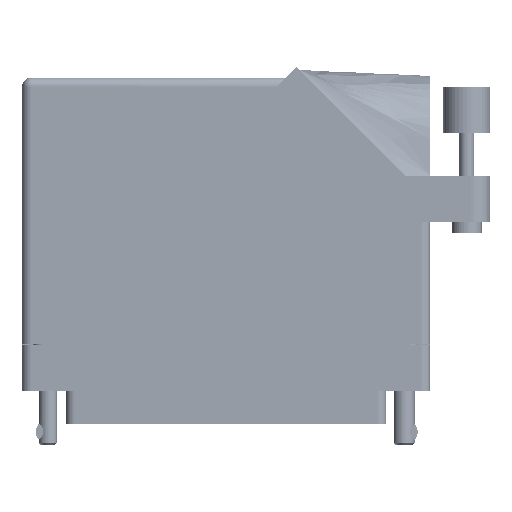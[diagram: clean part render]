
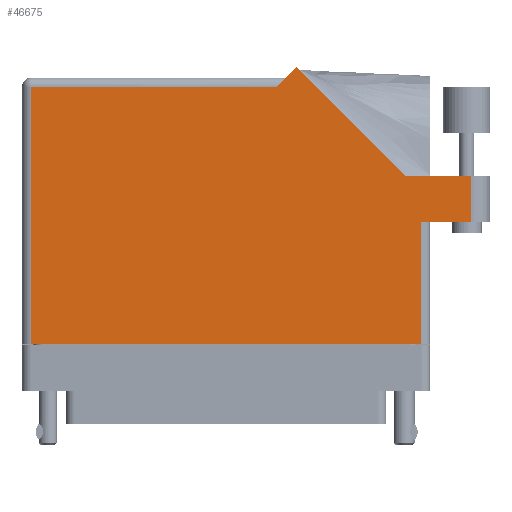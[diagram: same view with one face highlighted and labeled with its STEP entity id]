
A CAD part, front view. The second image highlights one B-rep face of the part: STEP entity #46675.
In plain terms, the highlighted face is planar.
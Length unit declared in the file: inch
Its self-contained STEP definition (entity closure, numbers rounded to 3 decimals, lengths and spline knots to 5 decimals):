
#30 = EDGE_CURVE ( 'NONE', #46746, #72187, #80173, .T. ) ;
#500 = EDGE_CURVE ( 'NONE', #21925, #56165, #10249, .T. ) ;
#1463 = CARTESIAN_POINT ( 'NONE',  ( -1.359, -0.1, 0.617 ) ) ;
#1577 = CARTESIAN_POINT ( 'NONE',  ( 0.399, 1.675, 0.617 ) ) ;
#2325 = DIRECTION ( 'NONE',  ( 1., 0., 0. ) ) ;
#2391 = CARTESIAN_POINT ( 'NONE',  ( 1.297, 0.715, 0.617 ) ) ;
#3229 = ORIENTED_EDGE ( 'NONE', *, *, #41724, .T. ) ;
#4679 = EDGE_CURVE ( 'NONE', #58465, #71421, #20613, .T. ) ;
#4954 = DIRECTION ( 'NONE',  ( 0., 1., 0. ) ) ;
#5821 = VECTOR ( 'NONE', #79149, 39.37008 ) ;
#6263 = DIRECTION ( 'NONE',  ( -1., 0., 0. ) ) ;
#9476 = PLANE ( 'NONE',  #22034 ) ;
#10249 = LINE ( 'NONE', #1463, #49826 ) ;
#11422 = CARTESIAN_POINT ( 'NONE',  ( -1.297, -0.1, 0.617 ) ) ;
#12130 = VECTOR ( 'NONE', #2325, 39.37008 ) ;
#12476 = CARTESIAN_POINT ( 'NONE',  ( 0.46971, 1.74571, 0.617 ) ) ;
#13965 = DIRECTION ( 'NONE',  ( 1., 0., 0. ) ) ;
#14523 = EDGE_CURVE ( 'NONE', #52448, #20298, #71336, .T. ) ;
#19420 = CARTESIAN_POINT ( 'NONE',  ( 1.19342, 1.022, 0.617 ) ) ;
#20298 = VERTEX_POINT ( 'NONE', #12476 ) ;
#20613 = LINE ( 'NONE', #63253, #82511 ) ;
#21925 = VERTEX_POINT ( 'NONE', #54139 ) ;
#22034 = AXIS2_PLACEMENT_3D ( 'NONE', #28182, #74313, #67791 ) ;
#25794 = EDGE_LOOP ( 'NONE', ( #36827, #33515, #50075, #69052, #67872, #47956, #40255, #82536, #3229 ) ) ;
#27352 = CARTESIAN_POINT ( 'NONE',  ( 1.297, 0.715, 0.617 ) ) ;
#27617 = LINE ( 'NONE', #11422, #52963 ) ;
#28182 = CARTESIAN_POINT ( 'NONE',  ( -1.359, 1.675, 0.617 ) ) ;
#29590 = CARTESIAN_POINT ( 'NONE',  ( 0.337, 1.613, 0.617 ) ) ;
#31802 = LINE ( 'NONE', #62358, #65240 ) ;
#33515 = ORIENTED_EDGE ( 'NONE', *, *, #4679, .T. ) ;
#33936 = EDGE_CURVE ( 'NONE', #41717, #58465, #78941, .T. ) ;
#35571 = CARTESIAN_POINT ( 'NONE',  ( 1.19342, 1.022, 0.617 ) ) ;
#36827 = ORIENTED_EDGE ( 'NONE', *, *, #33936, .T. ) ;
#36888 = EDGE_CURVE ( 'NONE', #71421, #52448, #31802, .T. ) ;
#36965 = VECTOR ( 'NONE', #42868, 39.37008 ) ;
#37316 = CARTESIAN_POINT ( 'NONE',  ( 1.297, -0.1, 0.617 ) ) ;
#38297 = CARTESIAN_POINT ( 'NONE',  ( -1.359, 1.613, 0.617 ) ) ;
#40255 = ORIENTED_EDGE ( 'NONE', *, *, #81030, .T. ) ;
#41669 = CARTESIAN_POINT ( 'NONE',  ( 1.634, 1.022, 0.617 ) ) ;
#41717 = VERTEX_POINT ( 'NONE', #2391 ) ;
#41724 = EDGE_CURVE ( 'NONE', #56165, #41717, #44319, .T. ) ;
#42868 = DIRECTION ( 'NONE',  ( -0.707, 0.707, 0. ) ) ;
#43730 = FACE_OUTER_BOUND ( 'NONE', #25794, .T. ) ;
#43926 = CARTESIAN_POINT ( 'NONE',  ( -1.297, 1.613, 0.617 ) ) ;
#44319 = LINE ( 'NONE', #27352, #5821 ) ;
#46675 = ADVANCED_FACE ( 'NONE', ( #43730 ), #9476, .F. ) ;
#46746 = VERTEX_POINT ( 'NONE', #29590 ) ;
#47373 = CARTESIAN_POINT ( 'NONE',  ( 1.359, 0.715, 0.617 ) ) ;
#47956 = ORIENTED_EDGE ( 'NONE', *, *, #30, .T. ) ;
#49826 = VECTOR ( 'NONE', #13965, 39.37008 ) ;
#50075 = ORIENTED_EDGE ( 'NONE', *, *, #36888, .T. ) ;
#50527 = LINE ( 'NONE', #1577, #82972 ) ;
#52448 = VERTEX_POINT ( 'NONE', #19420 ) ;
#52963 = VECTOR ( 'NONE', #83610, 39.37008 ) ;
#53813 = CARTESIAN_POINT ( 'NONE',  ( 1.634, 0.715, 0.617 ) ) ;
#54139 = CARTESIAN_POINT ( 'NONE',  ( -1.297, -0.1, 0.617 ) ) ;
#56165 = VERTEX_POINT ( 'NONE', #37316 ) ;
#58465 = VERTEX_POINT ( 'NONE', #53813 ) ;
#59454 = EDGE_CURVE ( 'NONE', #20298, #46746, #50527, .T. ) ;
#61788 = DIRECTION ( 'NONE',  ( -1., 0., 0. ) ) ;
#62358 = CARTESIAN_POINT ( 'NONE',  ( 1.759, 1.022, 0.617 ) ) ;
#63253 = CARTESIAN_POINT ( 'NONE',  ( 1.634, 1.022, 0.617 ) ) ;
#65240 = VECTOR ( 'NONE', #61788, 39.37008 ) ;
#67791 = DIRECTION ( 'NONE',  ( -1., 0., 0. ) ) ;
#67872 = ORIENTED_EDGE ( 'NONE', *, *, #59454, .T. ) ;
#69052 = ORIENTED_EDGE ( 'NONE', *, *, #14523, .T. ) ;
#71336 = LINE ( 'NONE', #35571, #36965 ) ;
#71421 = VERTEX_POINT ( 'NONE', #41669 ) ;
#72187 = VERTEX_POINT ( 'NONE', #43926 ) ;
#72350 = DIRECTION ( 'NONE',  ( -0.707, -0.707, 0. ) ) ;
#74313 = DIRECTION ( 'NONE',  ( 0., 0., -1. ) ) ;
#78941 = LINE ( 'NONE', #47373, #12130 ) ;
#79149 = DIRECTION ( 'NONE',  ( 0., 1., 0. ) ) ;
#80173 = LINE ( 'NONE', #38297, #82230 ) ;
#81030 = EDGE_CURVE ( 'NONE', #72187, #21925, #27617, .T. ) ;
#82230 = VECTOR ( 'NONE', #6263, 39.37008 ) ;
#82511 = VECTOR ( 'NONE', #4954, 39.37008 ) ;
#82536 = ORIENTED_EDGE ( 'NONE', *, *, #500, .T. ) ;
#82972 = VECTOR ( 'NONE', #72350, 39.37008 ) ;
#83610 = DIRECTION ( 'NONE',  ( 0., -1., 0. ) ) ;
